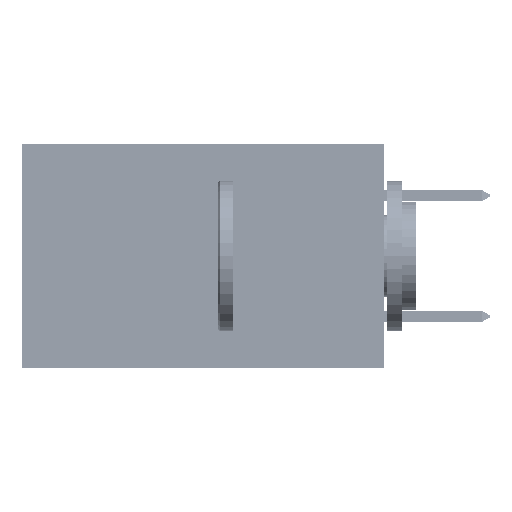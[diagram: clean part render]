
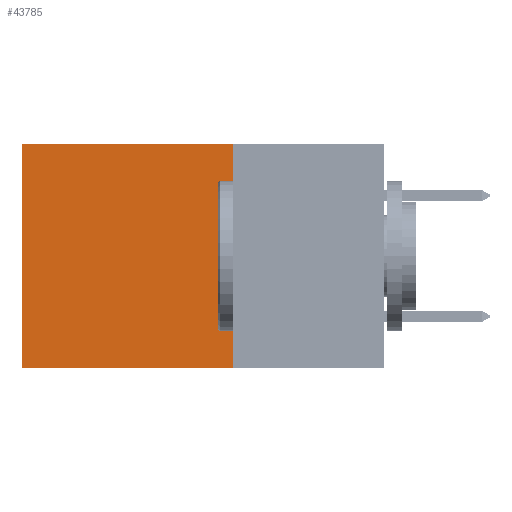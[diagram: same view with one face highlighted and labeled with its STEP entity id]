
A CAD part, left-side view. The second image highlights one B-rep face of the part: STEP entity #43785.
In plain terms, the highlighted planar face has unit normal (-1, 0, 0).
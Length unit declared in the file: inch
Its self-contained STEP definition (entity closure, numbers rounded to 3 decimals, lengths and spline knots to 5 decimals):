
#1 = ORIENTED_EDGE ( 'NONE', *, *, #2385, .F. ) ;
#1646 = ORIENTED_EDGE ( 'NONE', *, *, #37482, .F. ) ;
#2385 = EDGE_CURVE ( 'NONE', #42975, #42050, #44472, .T. ) ;
#3126 = CARTESIAN_POINT ( 'NONE',  ( 0.2875, 0.25, -0.37 ) ) ;
#4043 = EDGE_CURVE ( 'NONE', #46529, #42050, #22295, .T. ) ;
#5232 = CARTESIAN_POINT ( 'NONE',  ( 0.2875, 0.25, -0.37 ) ) ;
#9423 = EDGE_CURVE ( 'NONE', #27227, #46529, #48556, .T. ) ;
#11189 = EDGE_LOOP ( 'NONE', ( #17114, #1, #1646, #37208 ) ) ;
#14085 = VECTOR ( 'NONE', #35730, 39.37008 ) ;
#15774 = AXIS2_PLACEMENT_3D ( 'NONE', #49207, #45551, #22770 ) ;
#15868 = DIRECTION ( 'NONE',  ( 0., 0., -1. ) ) ;
#17114 = ORIENTED_EDGE ( 'NONE', *, *, #4043, .T. ) ;
#21761 = CARTESIAN_POINT ( 'NONE',  ( 0.2875, 0.25, 0. ) ) ;
#22295 = LINE ( 'NONE', #44914, #31200 ) ;
#22770 = DIRECTION ( 'NONE',  ( 0., 0., -1. ) ) ;
#27227 = VERTEX_POINT ( 'NONE', #40999 ) ;
#30193 = CARTESIAN_POINT ( 'NONE',  ( 0.2875, 0.6, 0. ) ) ;
#30200 = LINE ( 'NONE', #34850, #41466 ) ;
#31200 = VECTOR ( 'NONE', #41046, 39.37008 ) ;
#34850 = CARTESIAN_POINT ( 'NONE',  ( 0.2875, 0.25, 0. ) ) ;
#35730 = DIRECTION ( 'NONE',  ( 0., 1., 0. ) ) ;
#36032 = VECTOR ( 'NONE', #37020, 39.37008 ) ;
#37020 = DIRECTION ( 'NONE',  ( 0., 1., 0. ) ) ;
#37208 = ORIENTED_EDGE ( 'NONE', *, *, #9423, .T. ) ;
#37423 = FACE_OUTER_BOUND ( 'NONE', #11189, .T. ) ;
#37482 = EDGE_CURVE ( 'NONE', #27227, #42975, #30200, .T. ) ;
#40999 = CARTESIAN_POINT ( 'NONE',  ( 0.2875, 0.25, 0. ) ) ;
#41046 = DIRECTION ( 'NONE',  ( 0., 0., -1. ) ) ;
#41466 = VECTOR ( 'NONE', #15868, 39.37008 ) ;
#41674 = PLANE ( 'NONE',  #15774 ) ;
#42050 = VERTEX_POINT ( 'NONE', #47548 ) ;
#42975 = VERTEX_POINT ( 'NONE', #3126 ) ;
#43785 = ADVANCED_FACE ( 'NONE', ( #37423 ), #41674, .F. ) ;
#44472 = LINE ( 'NONE', #5232, #14085 ) ;
#44914 = CARTESIAN_POINT ( 'NONE',  ( 0.2875, 0.6, 0. ) ) ;
#45551 = DIRECTION ( 'NONE',  ( 1., 0., 0. ) ) ;
#46529 = VERTEX_POINT ( 'NONE', #30193 ) ;
#47548 = CARTESIAN_POINT ( 'NONE',  ( 0.2875, 0.6, -0.37 ) ) ;
#48556 = LINE ( 'NONE', #21761, #36032 ) ;
#49207 = CARTESIAN_POINT ( 'NONE',  ( 0.2875, 0.25, 0. ) ) ;
